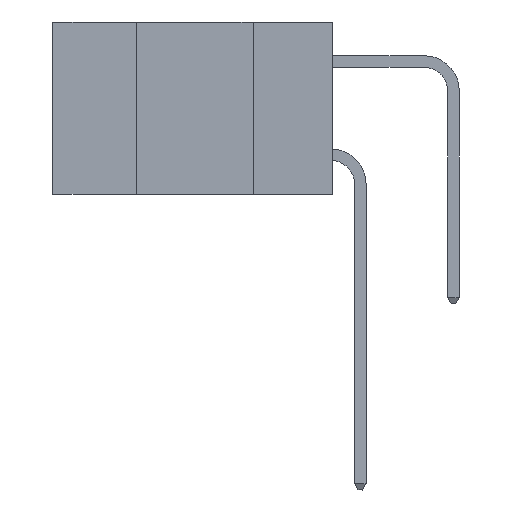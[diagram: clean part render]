
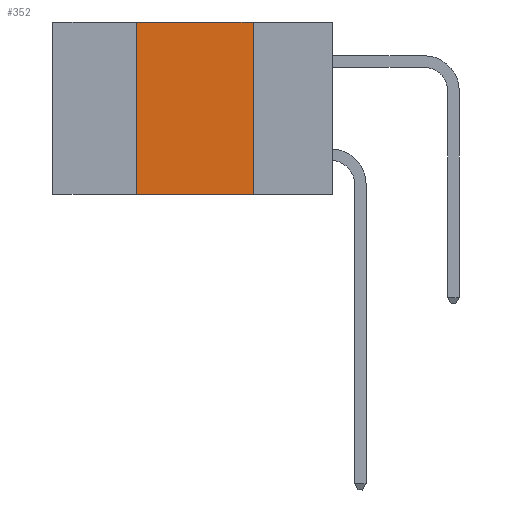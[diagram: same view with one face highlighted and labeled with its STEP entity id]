
A CAD part, left-side view. The second image highlights one B-rep face of the part: STEP entity #352.
In plain terms, the highlighted planar face has unit normal (-1, 0, 0).
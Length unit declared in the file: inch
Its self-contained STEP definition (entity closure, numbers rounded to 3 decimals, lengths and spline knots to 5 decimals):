
#38 = ORIENTED_EDGE ( 'NONE', *, *, #4385, .F. ) ;
#352 = ADVANCED_FACE ( 'NONE', ( #2287 ), #7377, .F. ) ;
#398 = CARTESIAN_POINT ( 'NONE',  ( 0., 0.6, 0. ) ) ;
#531 = DIRECTION ( 'NONE',  ( 0., -1., 0. ) ) ;
#806 = DIRECTION ( 'NONE',  ( 0., 0., 1. ) ) ;
#896 = CARTESIAN_POINT ( 'NONE',  ( 0., 0.42, 0. ) ) ;
#1196 = VERTEX_POINT ( 'NONE', #8753 ) ;
#1281 = VERTEX_POINT ( 'NONE', #11985 ) ;
#2172 = AXIS2_PLACEMENT_3D ( 'NONE', #398, #7463, #10588 ) ;
#2287 = FACE_OUTER_BOUND ( 'NONE', #6739, .T. ) ;
#2875 = ORIENTED_EDGE ( 'NONE', *, *, #6280, .F. ) ;
#3193 = ORIENTED_EDGE ( 'NONE', *, *, #10794, .F. ) ;
#3556 = VECTOR ( 'NONE', #806, 39.37008 ) ;
#4172 = VECTOR ( 'NONE', #9179, 39.37008 ) ;
#4385 = EDGE_CURVE ( 'NONE', #11360, #11750, #8996, .T. ) ;
#5055 = CARTESIAN_POINT ( 'NONE',  ( 0., 0.42, 0. ) ) ;
#5091 = CARTESIAN_POINT ( 'NONE',  ( 0., 0.6, -0.37 ) ) ;
#5350 = LINE ( 'NONE', #5583, #6610 ) ;
#5583 = CARTESIAN_POINT ( 'NONE',  ( 0., 0.17, 0. ) ) ;
#5773 = LINE ( 'NONE', #896, #3556 ) ;
#6280 = EDGE_CURVE ( 'NONE', #1196, #11360, #5773, .T. ) ;
#6514 = CARTESIAN_POINT ( 'NONE',  ( 0., 0.6, 0. ) ) ;
#6610 = VECTOR ( 'NONE', #11731, 39.37008 ) ;
#6739 = EDGE_LOOP ( 'NONE', ( #3193, #38, #2875, #7941 ) ) ;
#7161 = CARTESIAN_POINT ( 'NONE',  ( 0., 0.17, 0. ) ) ;
#7377 = PLANE ( 'NONE',  #2172 ) ;
#7463 = DIRECTION ( 'NONE',  ( 1., 0., 0. ) ) ;
#7534 = EDGE_CURVE ( 'NONE', #1196, #1281, #12390, .T. ) ;
#7941 = ORIENTED_EDGE ( 'NONE', *, *, #7534, .T. ) ;
#8753 = CARTESIAN_POINT ( 'NONE',  ( 0., 0.42, -0.37 ) ) ;
#8834 = VECTOR ( 'NONE', #531, 39.37008 ) ;
#8996 = LINE ( 'NONE', #6514, #8834 ) ;
#9179 = DIRECTION ( 'NONE',  ( 0., -1., 0. ) ) ;
#10588 = DIRECTION ( 'NONE',  ( 0., 0., -1. ) ) ;
#10794 = EDGE_CURVE ( 'NONE', #11750, #1281, #5350, .T. ) ;
#11360 = VERTEX_POINT ( 'NONE', #5055 ) ;
#11731 = DIRECTION ( 'NONE',  ( 0., 0., -1. ) ) ;
#11750 = VERTEX_POINT ( 'NONE', #7161 ) ;
#11985 = CARTESIAN_POINT ( 'NONE',  ( 0., 0.17, -0.37 ) ) ;
#12390 = LINE ( 'NONE', #5091, #4172 ) ;
